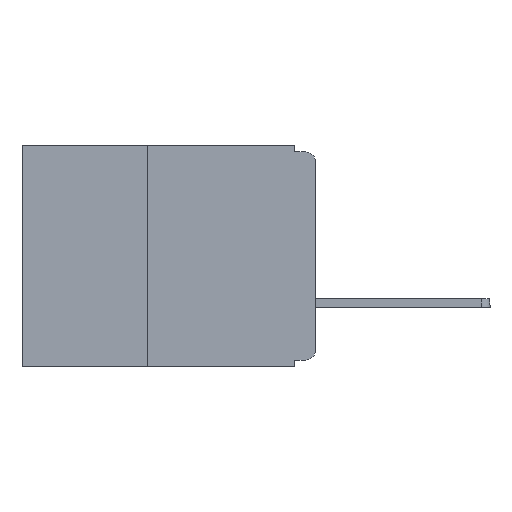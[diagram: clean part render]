
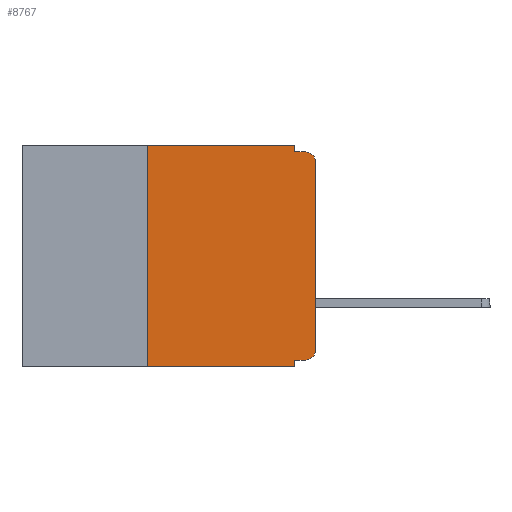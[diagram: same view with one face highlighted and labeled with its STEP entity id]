
A CAD part, left-side view. The second image highlights one B-rep face of the part: STEP entity #8767.
In plain terms, the highlighted planar face has unit normal (-1, 0, 0).
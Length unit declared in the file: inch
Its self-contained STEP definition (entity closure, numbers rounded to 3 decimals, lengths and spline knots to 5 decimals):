
#17 = VERTEX_POINT ( 'NONE', #1750 ) ;
#702 = EDGE_CURVE ( 'NONE', #17, #2907, #1482, .T. ) ;
#728 = LINE ( 'NONE', #14222, #7259 ) ;
#877 = EDGE_CURVE ( 'NONE', #10693, #11328, #11216, .T. ) ;
#1068 = VECTOR ( 'NONE', #7280, 39.37008 ) ;
#1284 = EDGE_CURVE ( 'NONE', #10037, #8243, #10089, .T. ) ;
#1361 = CARTESIAN_POINT ( 'NONE',  ( 0., 0., -0.01 ) ) ;
#1482 = LINE ( 'NONE', #7052, #1068 ) ;
#1541 = EDGE_CURVE ( 'NONE', #2907, #11328, #9902, .T. ) ;
#1555 = CARTESIAN_POINT ( 'NONE',  ( 0., 0.031, 0. ) ) ;
#1750 = CARTESIAN_POINT ( 'NONE',  ( 0., 0., -0.305 ) ) ;
#1772 = EDGE_CURVE ( 'NONE', #10037, #17, #3127, .T. ) ;
#2011 = ORIENTED_EDGE ( 'NONE', *, *, #4703, .F. ) ;
#2212 = LINE ( 'NONE', #13278, #6098 ) ;
#2251 = EDGE_CURVE ( 'NONE', #8858, #8327, #12507, .T. ) ;
#2486 = VECTOR ( 'NONE', #2727, 39.37008 ) ;
#2725 = DIRECTION ( 'NONE',  ( 0., -1., 0. ) ) ;
#2727 = DIRECTION ( 'NONE',  ( 0., -1., 0. ) ) ;
#2907 = VERTEX_POINT ( 'NONE', #8198 ) ;
#2943 = DIRECTION ( 'NONE',  ( 0., 0., -1. ) ) ;
#3027 = ORIENTED_EDGE ( 'NONE', *, *, #702, .T. ) ;
#3127 = CIRCLE ( 'NONE', #5211, 0.015 ) ;
#3826 = CARTESIAN_POINT ( 'NONE',  ( 0., 0.015, -0.025 ) ) ;
#4546 = CARTESIAN_POINT ( 'NONE',  ( 0., 0., -0.32 ) ) ;
#4569 = EDGE_CURVE ( 'NONE', #8327, #10693, #7993, .T. ) ;
#4595 = EDGE_CURVE ( 'NONE', #13504, #8858, #728, .T. ) ;
#4643 = EDGE_CURVE ( 'NONE', #13504, #14151, #15370, .T. ) ;
#4703 = EDGE_CURVE ( 'NONE', #8243, #14151, #2212, .T. ) ;
#4733 = VECTOR ( 'NONE', #14283, 39.37008 ) ;
#5211 = AXIS2_PLACEMENT_3D ( 'NONE', #5589, #5509, #2943 ) ;
#5509 = DIRECTION ( 'NONE',  ( -1., 0., 0. ) ) ;
#5589 = CARTESIAN_POINT ( 'NONE',  ( 0., 0.015, -0.305 ) ) ;
#6098 = VECTOR ( 'NONE', #13293, 39.37008 ) ;
#6300 = ORIENTED_EDGE ( 'NONE', *, *, #2251, .F. ) ;
#6500 = CARTESIAN_POINT ( 'NONE',  ( 0., 0.437, 0. ) ) ;
#6715 = CARTESIAN_POINT ( 'NONE',  ( 0., 0.25, 0. ) ) ;
#6868 = ORIENTED_EDGE ( 'NONE', *, *, #1541, .T. ) ;
#7052 = CARTESIAN_POINT ( 'NONE',  ( 0., 0., 0. ) ) ;
#7259 = VECTOR ( 'NONE', #14208, 39.37008 ) ;
#7280 = DIRECTION ( 'NONE',  ( 0., 0., 1. ) ) ;
#7700 = DIRECTION ( 'NONE',  ( 1., 0., 0. ) ) ;
#7939 = AXIS2_PLACEMENT_3D ( 'NONE', #3826, #12034, #12402 ) ;
#7993 = LINE ( 'NONE', #14384, #4733 ) ;
#8092 = VECTOR ( 'NONE', #2725, 39.37008 ) ;
#8198 = CARTESIAN_POINT ( 'NONE',  ( 0., 0., -0.025 ) ) ;
#8243 = VERTEX_POINT ( 'NONE', #11291 ) ;
#8327 = VERTEX_POINT ( 'NONE', #1555 ) ;
#8525 = ORIENTED_EDGE ( 'NONE', *, *, #4595, .F. ) ;
#8581 = FACE_OUTER_BOUND ( 'NONE', #10568, .T. ) ;
#8707 = ORIENTED_EDGE ( 'NONE', *, *, #4569, .F. ) ;
#8767 = ADVANCED_FACE ( 'NONE', ( #8581 ), #13294, .F. ) ;
#8858 = VERTEX_POINT ( 'NONE', #6715 ) ;
#8924 = ORIENTED_EDGE ( 'NONE', *, *, #4643, .T. ) ;
#9855 = ORIENTED_EDGE ( 'NONE', *, *, #1772, .T. ) ;
#9902 = CIRCLE ( 'NONE', #7939, 0.015 ) ;
#10037 = VERTEX_POINT ( 'NONE', #10252 ) ;
#10089 = LINE ( 'NONE', #4546, #12687 ) ;
#10252 = CARTESIAN_POINT ( 'NONE',  ( 0., 0.015, -0.32 ) ) ;
#10568 = EDGE_LOOP ( 'NONE', ( #3027, #6868, #13240, #8707, #6300, #8525, #8924, #2011, #14590, #9855 ) ) ;
#10693 = VERTEX_POINT ( 'NONE', #11532 ) ;
#10980 = CARTESIAN_POINT ( 'NONE',  ( 0., 0.031, -0.33 ) ) ;
#11216 = LINE ( 'NONE', #1361, #8092 ) ;
#11291 = CARTESIAN_POINT ( 'NONE',  ( 0., 0.031, -0.32 ) ) ;
#11328 = VERTEX_POINT ( 'NONE', #12503 ) ;
#11532 = CARTESIAN_POINT ( 'NONE',  ( 0., 0.031, -0.01 ) ) ;
#11757 = AXIS2_PLACEMENT_3D ( 'NONE', #6500, #7700, #15384 ) ;
#12034 = DIRECTION ( 'NONE',  ( -1., 0., 0. ) ) ;
#12075 = CARTESIAN_POINT ( 'NONE',  ( 0., 0.437, 0. ) ) ;
#12402 = DIRECTION ( 'NONE',  ( 0., 0., -1. ) ) ;
#12503 = CARTESIAN_POINT ( 'NONE',  ( 0., 0.015, -0.01 ) ) ;
#12507 = LINE ( 'NONE', #12075, #2486 ) ;
#12605 = DIRECTION ( 'NONE',  ( 0., 1., 0. ) ) ;
#12614 = VECTOR ( 'NONE', #13880, 39.37008 ) ;
#12687 = VECTOR ( 'NONE', #12605, 39.37008 ) ;
#13240 = ORIENTED_EDGE ( 'NONE', *, *, #877, .F. ) ;
#13278 = CARTESIAN_POINT ( 'NONE',  ( 0., 0.031, -0.33 ) ) ;
#13293 = DIRECTION ( 'NONE',  ( 0., 0., -1. ) ) ;
#13294 = PLANE ( 'NONE',  #11757 ) ;
#13447 = CARTESIAN_POINT ( 'NONE',  ( 0., 0.25, -0.33 ) ) ;
#13504 = VERTEX_POINT ( 'NONE', #13447 ) ;
#13812 = CARTESIAN_POINT ( 'NONE',  ( 0., 0.437, -0.33 ) ) ;
#13880 = DIRECTION ( 'NONE',  ( 0., -1., 0. ) ) ;
#14151 = VERTEX_POINT ( 'NONE', #10980 ) ;
#14208 = DIRECTION ( 'NONE',  ( 0., 0., 1. ) ) ;
#14222 = CARTESIAN_POINT ( 'NONE',  ( 0., 0.25, -0.33 ) ) ;
#14283 = DIRECTION ( 'NONE',  ( 0., 0., -1. ) ) ;
#14384 = CARTESIAN_POINT ( 'NONE',  ( 0., 0.031, 0. ) ) ;
#14590 = ORIENTED_EDGE ( 'NONE', *, *, #1284, .F. ) ;
#15370 = LINE ( 'NONE', #13812, #12614 ) ;
#15384 = DIRECTION ( 'NONE',  ( 0., 0., -1. ) ) ;
